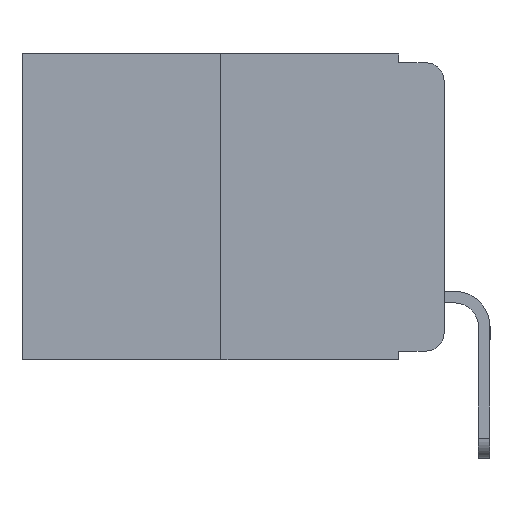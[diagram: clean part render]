
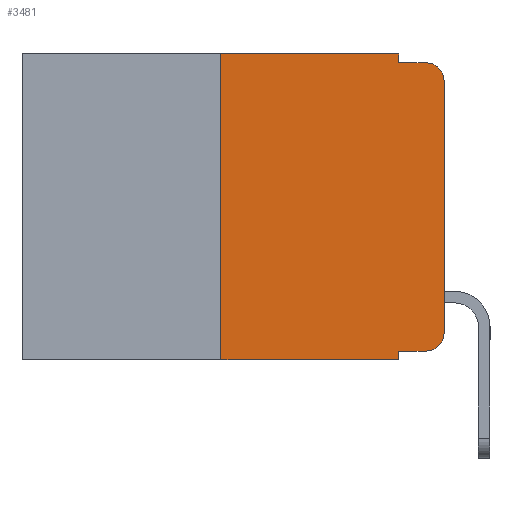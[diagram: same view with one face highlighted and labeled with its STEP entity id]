
A CAD part, left-side view. The second image highlights one B-rep face of the part: STEP entity #3481.
In plain terms, the highlighted planar face has unit normal (-1, 0, 0).
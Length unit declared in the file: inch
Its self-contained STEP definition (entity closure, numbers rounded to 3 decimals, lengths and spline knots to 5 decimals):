
#219 = CARTESIAN_POINT ( 'NONE',  ( 0., 0.051, 0. ) ) ;
#341 = CIRCLE ( 'NONE', #1516, 0.02 ) ;
#480 = ORIENTED_EDGE ( 'NONE', *, *, #3339, .F. ) ;
#865 = VECTOR ( 'NONE', #5722, 39.37008 ) ;
#1069 = VERTEX_POINT ( 'NONE', #3277 ) ;
#1141 = VECTOR ( 'NONE', #1835, 39.37008 ) ;
#1190 = VERTEX_POINT ( 'NONE', #4432 ) ;
#1289 = ORIENTED_EDGE ( 'NONE', *, *, #1314, .T. ) ;
#1314 = EDGE_CURVE ( 'NONE', #1506, #2727, #8255, .T. ) ;
#1353 = ORIENTED_EDGE ( 'NONE', *, *, #9334, .F. ) ;
#1506 = VERTEX_POINT ( 'NONE', #6176 ) ;
#1516 = AXIS2_PLACEMENT_3D ( 'NONE', #4263, #4235, #3399 ) ;
#1553 = VERTEX_POINT ( 'NONE', #6971 ) ;
#1579 = DIRECTION ( 'NONE',  ( 1., 0., 0. ) ) ;
#1835 = DIRECTION ( 'NONE',  ( 0., 0., -1. ) ) ;
#1855 = CARTESIAN_POINT ( 'NONE',  ( 0., 0.051, -0.333 ) ) ;
#2111 = ORIENTED_EDGE ( 'NONE', *, *, #3520, .T. ) ;
#2130 = ORIENTED_EDGE ( 'NONE', *, *, #5908, .T. ) ;
#2203 = DIRECTION ( 'NONE',  ( -1., 0., 0. ) ) ;
#2494 = ORIENTED_EDGE ( 'NONE', *, *, #4545, .F. ) ;
#2727 = VERTEX_POINT ( 'NONE', #9145 ) ;
#2892 = AXIS2_PLACEMENT_3D ( 'NONE', #3413, #1579, #10864 ) ;
#3107 = LINE ( 'NONE', #9901, #9154 ) ;
#3277 = CARTESIAN_POINT ( 'NONE',  ( 0., 0., -0.03 ) ) ;
#3317 = EDGE_CURVE ( 'NONE', #6976, #1190, #4499, .T. ) ;
#3339 = EDGE_CURVE ( 'NONE', #5421, #6976, #6218, .T. ) ;
#3399 = DIRECTION ( 'NONE',  ( 0., 0., -1. ) ) ;
#3413 = CARTESIAN_POINT ( 'NONE',  ( 0., 0.473, 0. ) ) ;
#3481 = ADVANCED_FACE ( 'NONE', ( #8097 ), #10630, .F. ) ;
#3520 = EDGE_CURVE ( 'NONE', #2727, #4329, #341, .T. ) ;
#3547 = CARTESIAN_POINT ( 'NONE',  ( 0., 0.473, 0. ) ) ;
#3914 = LINE ( 'NONE', #7195, #1141 ) ;
#4081 = LINE ( 'NONE', #6315, #8303 ) ;
#4206 = ORIENTED_EDGE ( 'NONE', *, *, #7810, .T. ) ;
#4220 = VECTOR ( 'NONE', #6189, 39.37008 ) ;
#4235 = DIRECTION ( 'NONE',  ( -1., 0., 0. ) ) ;
#4263 = CARTESIAN_POINT ( 'NONE',  ( 0., 0.02, -0.313 ) ) ;
#4269 = CARTESIAN_POINT ( 'NONE',  ( 0., 0.25, -0.343 ) ) ;
#4329 = VERTEX_POINT ( 'NONE', #10059 ) ;
#4397 = DIRECTION ( 'NONE',  ( 0., 0., 1. ) ) ;
#4432 = CARTESIAN_POINT ( 'NONE',  ( 0., 0.02, -0.01 ) ) ;
#4499 = LINE ( 'NONE', #6912, #4220 ) ;
#4545 = EDGE_CURVE ( 'NONE', #10705, #1553, #4081, .T. ) ;
#4717 = DIRECTION ( 'NONE',  ( 0., -1., 0. ) ) ;
#5253 = ORIENTED_EDGE ( 'NONE', *, *, #10665, .T. ) ;
#5421 = VERTEX_POINT ( 'NONE', #219 ) ;
#5653 = EDGE_CURVE ( 'NONE', #1506, #8403, #3914, .T. ) ;
#5722 = DIRECTION ( 'NONE',  ( 0., 0., -1. ) ) ;
#5822 = CIRCLE ( 'NONE', #7923, 0.02 ) ;
#5908 = EDGE_CURVE ( 'NONE', #4329, #1069, #3107, .T. ) ;
#6176 = CARTESIAN_POINT ( 'NONE',  ( 0., 0.051, -0.333 ) ) ;
#6177 = DIRECTION ( 'NONE',  ( 0., -1., 0. ) ) ;
#6189 = DIRECTION ( 'NONE',  ( 0., -1., 0. ) ) ;
#6218 = LINE ( 'NONE', #8948, #865 ) ;
#6315 = CARTESIAN_POINT ( 'NONE',  ( 0., 0.25, 0. ) ) ;
#6410 = DIRECTION ( 'NONE',  ( 0., 0., 1. ) ) ;
#6568 = CARTESIAN_POINT ( 'NONE',  ( 0., 0.051, -0.343 ) ) ;
#6724 = VECTOR ( 'NONE', #6177, 39.37008 ) ;
#6889 = CARTESIAN_POINT ( 'NONE',  ( 0., 0.473, -0.343 ) ) ;
#6912 = CARTESIAN_POINT ( 'NONE',  ( 0., 0.051, -0.01 ) ) ;
#6920 = ORIENTED_EDGE ( 'NONE', *, *, #3317, .F. ) ;
#6971 = CARTESIAN_POINT ( 'NONE',  ( 0., 0.25, 0. ) ) ;
#6976 = VERTEX_POINT ( 'NONE', #6996 ) ;
#6996 = CARTESIAN_POINT ( 'NONE',  ( 0., 0.051, -0.01 ) ) ;
#7195 = CARTESIAN_POINT ( 'NONE',  ( 0., 0.051, 0. ) ) ;
#7486 = CARTESIAN_POINT ( 'NONE',  ( 0., 0.02, -0.03 ) ) ;
#7810 = EDGE_CURVE ( 'NONE', #10705, #8403, #8725, .T. ) ;
#7923 = AXIS2_PLACEMENT_3D ( 'NONE', #7486, #2203, #8228 ) ;
#8097 = FACE_OUTER_BOUND ( 'NONE', #9037, .T. ) ;
#8228 = DIRECTION ( 'NONE',  ( 0., 0., -1. ) ) ;
#8255 = LINE ( 'NONE', #1855, #10073 ) ;
#8303 = VECTOR ( 'NONE', #6410, 39.37008 ) ;
#8403 = VERTEX_POINT ( 'NONE', #6568 ) ;
#8410 = DIRECTION ( 'NONE',  ( 0., -1., 0. ) ) ;
#8725 = LINE ( 'NONE', #6889, #6724 ) ;
#8948 = CARTESIAN_POINT ( 'NONE',  ( 0., 0.051, 0. ) ) ;
#9037 = EDGE_LOOP ( 'NONE', ( #2130, #5253, #6920, #480, #1353, #2494, #4206, #9362, #1289, #2111 ) ) ;
#9145 = CARTESIAN_POINT ( 'NONE',  ( 0., 0.02, -0.333 ) ) ;
#9154 = VECTOR ( 'NONE', #4397, 39.37008 ) ;
#9334 = EDGE_CURVE ( 'NONE', #1553, #5421, #11183, .T. ) ;
#9362 = ORIENTED_EDGE ( 'NONE', *, *, #5653, .F. ) ;
#9433 = VECTOR ( 'NONE', #8410, 39.37008 ) ;
#9901 = CARTESIAN_POINT ( 'NONE',  ( 0., 0., 0. ) ) ;
#10059 = CARTESIAN_POINT ( 'NONE',  ( 0., 0., -0.313 ) ) ;
#10073 = VECTOR ( 'NONE', #4717, 39.37008 ) ;
#10630 = PLANE ( 'NONE',  #2892 ) ;
#10665 = EDGE_CURVE ( 'NONE', #1069, #1190, #5822, .T. ) ;
#10705 = VERTEX_POINT ( 'NONE', #4269 ) ;
#10864 = DIRECTION ( 'NONE',  ( 0., 0., -1. ) ) ;
#11183 = LINE ( 'NONE', #3547, #9433 ) ;
